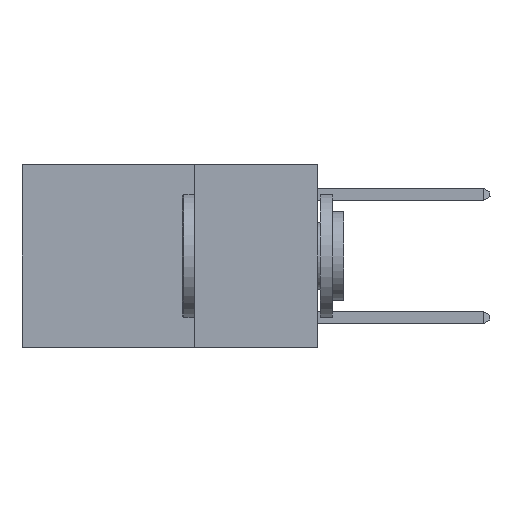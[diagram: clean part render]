
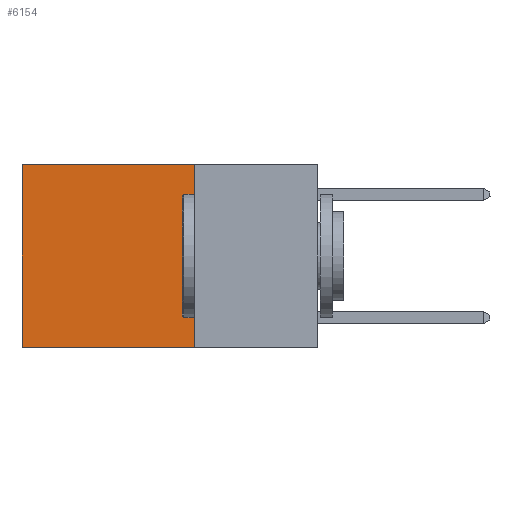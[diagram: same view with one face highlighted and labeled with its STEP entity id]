
A CAD part, left-side view. The second image highlights one B-rep face of the part: STEP entity #6154.
In plain terms, the highlighted planar face has unit normal (-1, 0, 0).
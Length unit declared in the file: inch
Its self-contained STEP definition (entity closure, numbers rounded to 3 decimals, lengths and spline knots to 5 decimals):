
#493 = DIRECTION ( 'NONE',  ( 0., 0., -1. ) ) ;
#511 = DIRECTION ( 'NONE',  ( 0., 1., 0. ) ) ;
#824 = CARTESIAN_POINT ( 'NONE',  ( 0.2625, 0.25, 0. ) ) ;
#1940 = DIRECTION ( 'NONE',  ( 0., 0., -1. ) ) ;
#2116 = EDGE_CURVE ( 'NONE', #10206, #4333, #12343, .T. ) ;
#2301 = VECTOR ( 'NONE', #12409, 39.37008 ) ;
#2486 = PLANE ( 'NONE',  #10243 ) ;
#3485 = EDGE_LOOP ( 'NONE', ( #8632, #7582, #8528, #7215 ) ) ;
#3861 = CARTESIAN_POINT ( 'NONE',  ( 0.2625, 0.6, 0. ) ) ;
#4333 = VERTEX_POINT ( 'NONE', #10353 ) ;
#4571 = DIRECTION ( 'NONE',  ( 1., 0., 0. ) ) ;
#4776 = CARTESIAN_POINT ( 'NONE',  ( 0.2625, 0.25, 0. ) ) ;
#5067 = CARTESIAN_POINT ( 'NONE',  ( 0.2625, 0.6, 0. ) ) ;
#5352 = EDGE_CURVE ( 'NONE', #10748, #10206, #11505, .T. ) ;
#5571 = VECTOR ( 'NONE', #10063, 39.37008 ) ;
#6154 = ADVANCED_FACE ( 'NONE', ( #10533 ), #2486, .F. ) ;
#6678 = VECTOR ( 'NONE', #1940, 39.37008 ) ;
#7215 = ORIENTED_EDGE ( 'NONE', *, *, #5352, .T. ) ;
#7582 = ORIENTED_EDGE ( 'NONE', *, *, #11244, .F. ) ;
#8454 = CARTESIAN_POINT ( 'NONE',  ( 0.2625, 0.25, -0.37 ) ) ;
#8528 = ORIENTED_EDGE ( 'NONE', *, *, #11537, .F. ) ;
#8632 = ORIENTED_EDGE ( 'NONE', *, *, #2116, .T. ) ;
#9146 = VERTEX_POINT ( 'NONE', #12541 ) ;
#9672 = CARTESIAN_POINT ( 'NONE',  ( 0.2625, 0.25, 0. ) ) ;
#9826 = LINE ( 'NONE', #824, #6678 ) ;
#10063 = DIRECTION ( 'NONE',  ( 0., 0., -1. ) ) ;
#10206 = VERTEX_POINT ( 'NONE', #3861 ) ;
#10243 = AXIS2_PLACEMENT_3D ( 'NONE', #9672, #4571, #493 ) ;
#10353 = CARTESIAN_POINT ( 'NONE',  ( 0.2625, 0.6, -0.37 ) ) ;
#10376 = CARTESIAN_POINT ( 'NONE',  ( 0.2625, 0.25, 0. ) ) ;
#10533 = FACE_OUTER_BOUND ( 'NONE', #3485, .T. ) ;
#10748 = VERTEX_POINT ( 'NONE', #10376 ) ;
#11244 = EDGE_CURVE ( 'NONE', #9146, #4333, #11544, .T. ) ;
#11505 = LINE ( 'NONE', #4776, #2301 ) ;
#11537 = EDGE_CURVE ( 'NONE', #10748, #9146, #9826, .T. ) ;
#11544 = LINE ( 'NONE', #8454, #11708 ) ;
#11708 = VECTOR ( 'NONE', #511, 39.37008 ) ;
#12343 = LINE ( 'NONE', #5067, #5571 ) ;
#12409 = DIRECTION ( 'NONE',  ( 0., 1., 0. ) ) ;
#12541 = CARTESIAN_POINT ( 'NONE',  ( 0.2625, 0.25, -0.37 ) ) ;
